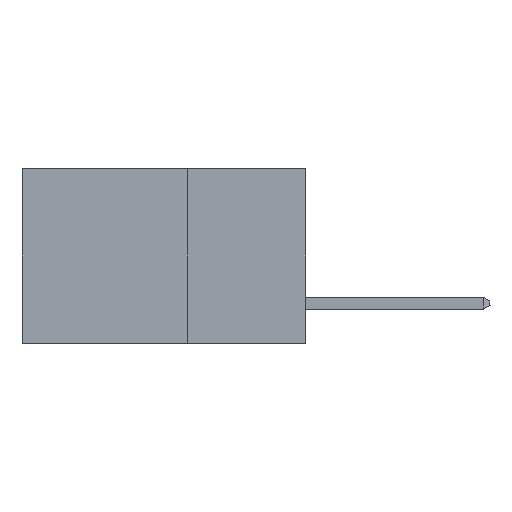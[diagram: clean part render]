
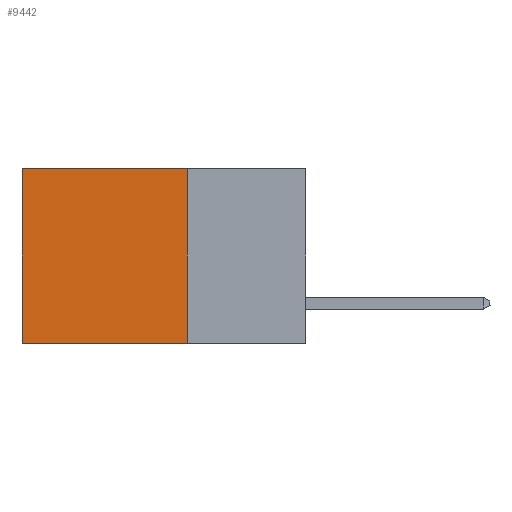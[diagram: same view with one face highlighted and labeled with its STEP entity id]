
A CAD part, left-side view. The second image highlights one B-rep face of the part: STEP entity #9442.
In plain terms, the highlighted planar face has unit normal (-1, 0, 0).
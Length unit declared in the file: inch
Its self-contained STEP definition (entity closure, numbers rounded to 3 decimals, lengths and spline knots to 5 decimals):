
#411 = EDGE_LOOP ( 'NONE', ( #1922, #3571, #4078, #11068 ) ) ;
#1427 = DIRECTION ( 'NONE',  ( 0., 0., -1. ) ) ;
#1893 = LINE ( 'NONE', #3313, #13128 ) ;
#1922 = ORIENTED_EDGE ( 'NONE', *, *, #9093, .T. ) ;
#2017 = CARTESIAN_POINT ( 'NONE',  ( 0.298, 0.6, 0. ) ) ;
#2189 = CARTESIAN_POINT ( 'NONE',  ( 0.298, 0.25, 0. ) ) ;
#2937 = VECTOR ( 'NONE', #4388, 39.37008 ) ;
#3218 = DIRECTION ( 'NONE',  ( 0., 1., 0. ) ) ;
#3313 = CARTESIAN_POINT ( 'NONE',  ( 0.298, 0.25, -0.37 ) ) ;
#3571 = ORIENTED_EDGE ( 'NONE', *, *, #7958, .F. ) ;
#3865 = EDGE_CURVE ( 'NONE', #11726, #13359, #12655, .T. ) ;
#3891 = VECTOR ( 'NONE', #4515, 39.37008 ) ;
#3908 = CARTESIAN_POINT ( 'NONE',  ( 0.298, 0.25, -0.37 ) ) ;
#4078 = ORIENTED_EDGE ( 'NONE', *, *, #13648, .F. ) ;
#4388 = DIRECTION ( 'NONE',  ( 0., 1., 0. ) ) ;
#4515 = DIRECTION ( 'NONE',  ( 0., 0., -1. ) ) ;
#4824 = CARTESIAN_POINT ( 'NONE',  ( 0.298, 0.6, -0.37 ) ) ;
#4983 = PLANE ( 'NONE',  #9571 ) ;
#6347 = VERTEX_POINT ( 'NONE', #3908 ) ;
#7291 = CARTESIAN_POINT ( 'NONE',  ( 0.298, 0.6, 0. ) ) ;
#7523 = LINE ( 'NONE', #11222, #10070 ) ;
#7681 = VERTEX_POINT ( 'NONE', #4824 ) ;
#7958 = EDGE_CURVE ( 'NONE', #6347, #7681, #1893, .T. ) ;
#8174 = CARTESIAN_POINT ( 'NONE',  ( 0.298, 0.25, 0. ) ) ;
#8229 = DIRECTION ( 'NONE',  ( 0., 0., -1. ) ) ;
#9093 = EDGE_CURVE ( 'NONE', #13359, #7681, #9179, .T. ) ;
#9179 = LINE ( 'NONE', #2017, #3891 ) ;
#9442 = ADVANCED_FACE ( 'NONE', ( #11206 ), #4983, .F. ) ;
#9571 = AXIS2_PLACEMENT_3D ( 'NONE', #8174, #12597, #8229 ) ;
#10070 = VECTOR ( 'NONE', #1427, 39.37008 ) ;
#11068 = ORIENTED_EDGE ( 'NONE', *, *, #3865, .T. ) ;
#11206 = FACE_OUTER_BOUND ( 'NONE', #411, .T. ) ;
#11222 = CARTESIAN_POINT ( 'NONE',  ( 0.298, 0.25, 0. ) ) ;
#11726 = VERTEX_POINT ( 'NONE', #13106 ) ;
#12597 = DIRECTION ( 'NONE',  ( 1., 0., 0. ) ) ;
#12655 = LINE ( 'NONE', #2189, #2937 ) ;
#13106 = CARTESIAN_POINT ( 'NONE',  ( 0.298, 0.25, 0. ) ) ;
#13128 = VECTOR ( 'NONE', #3218, 39.37008 ) ;
#13359 = VERTEX_POINT ( 'NONE', #7291 ) ;
#13648 = EDGE_CURVE ( 'NONE', #11726, #6347, #7523, .T. ) ;
